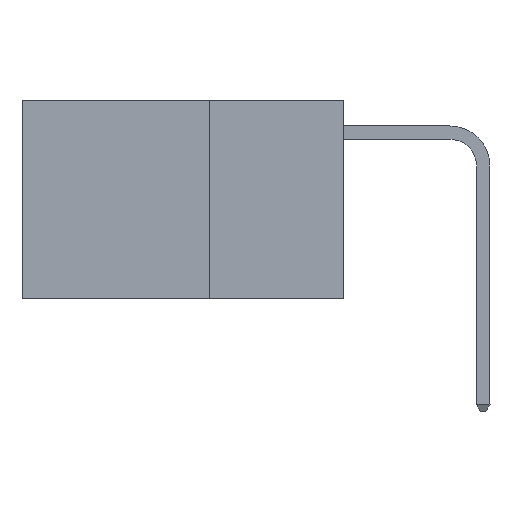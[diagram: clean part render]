
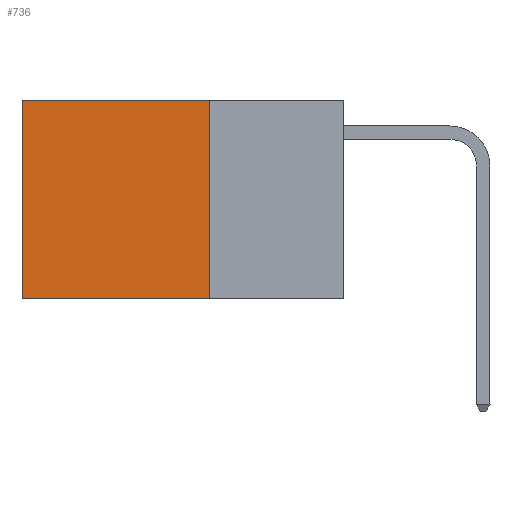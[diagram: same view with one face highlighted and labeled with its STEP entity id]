
A CAD part, left-side view. The second image highlights one B-rep face of the part: STEP entity #736.
In plain terms, the highlighted planar face has unit normal (-1, 0, 0).
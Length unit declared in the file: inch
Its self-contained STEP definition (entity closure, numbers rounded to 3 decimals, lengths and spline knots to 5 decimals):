
#532 = DIRECTION ( 'NONE',  ( 0., 0., -1. ) ) ;
#736 = ADVANCED_FACE ( 'NONE', ( #15885 ), #7297, .F. ) ;
#1349 = CARTESIAN_POINT ( 'NONE',  ( 0.2625, 0.25, 0. ) ) ;
#1964 = EDGE_CURVE ( 'NONE', #10321, #11434, #21722, .T. ) ;
#2044 = CARTESIAN_POINT ( 'NONE',  ( 0.2625, 0.25, -0.37 ) ) ;
#2148 = VERTEX_POINT ( 'NONE', #2044 ) ;
#2598 = CARTESIAN_POINT ( 'NONE',  ( 0.2625, 0.6, 0. ) ) ;
#3724 = VECTOR ( 'NONE', #16646, 39.37008 ) ;
#4122 = VERTEX_POINT ( 'NONE', #23103 ) ;
#6244 = LINE ( 'NONE', #12628, #3724 ) ;
#6769 = DIRECTION ( 'NONE',  ( 0., 0., -1. ) ) ;
#7297 = PLANE ( 'NONE',  #14244 ) ;
#8286 = DIRECTION ( 'NONE',  ( 0., 1., 0. ) ) ;
#10321 = VERTEX_POINT ( 'NONE', #18820 ) ;
#11434 = VERTEX_POINT ( 'NONE', #18121 ) ;
#12608 = ORIENTED_EDGE ( 'NONE', *, *, #15217, .T. ) ;
#12628 = CARTESIAN_POINT ( 'NONE',  ( 0.2625, 0.25, 0. ) ) ;
#13954 = DIRECTION ( 'NONE',  ( 1., 0., 0. ) ) ;
#14244 = AXIS2_PLACEMENT_3D ( 'NONE', #1349, #13954, #19773 ) ;
#15217 = EDGE_CURVE ( 'NONE', #4122, #10321, #6244, .T. ) ;
#15885 = FACE_OUTER_BOUND ( 'NONE', #16530, .T. ) ;
#15963 = EDGE_CURVE ( 'NONE', #2148, #11434, #17008, .T. ) ;
#16530 = EDGE_LOOP ( 'NONE', ( #24237, #25617, #23833, #12608 ) ) ;
#16646 = DIRECTION ( 'NONE',  ( 0., 1., 0. ) ) ;
#17008 = LINE ( 'NONE', #25458, #25921 ) ;
#18121 = CARTESIAN_POINT ( 'NONE',  ( 0.2625, 0.6, -0.37 ) ) ;
#18820 = CARTESIAN_POINT ( 'NONE',  ( 0.2625, 0.6, 0. ) ) ;
#19118 = CARTESIAN_POINT ( 'NONE',  ( 0.2625, 0.25, 0. ) ) ;
#19773 = DIRECTION ( 'NONE',  ( 0., 0., -1. ) ) ;
#21722 = LINE ( 'NONE', #2598, #26388 ) ;
#22753 = VECTOR ( 'NONE', #6769, 39.37008 ) ;
#23103 = CARTESIAN_POINT ( 'NONE',  ( 0.2625, 0.25, 0. ) ) ;
#23299 = EDGE_CURVE ( 'NONE', #4122, #2148, #25753, .T. ) ;
#23833 = ORIENTED_EDGE ( 'NONE', *, *, #23299, .F. ) ;
#24237 = ORIENTED_EDGE ( 'NONE', *, *, #1964, .T. ) ;
#25458 = CARTESIAN_POINT ( 'NONE',  ( 0.2625, 0.25, -0.37 ) ) ;
#25617 = ORIENTED_EDGE ( 'NONE', *, *, #15963, .F. ) ;
#25753 = LINE ( 'NONE', #19118, #22753 ) ;
#25921 = VECTOR ( 'NONE', #8286, 39.37008 ) ;
#26388 = VECTOR ( 'NONE', #532, 39.37008 ) ;
